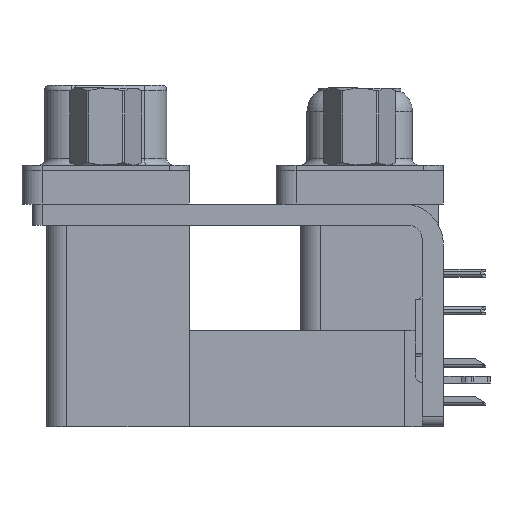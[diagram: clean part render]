
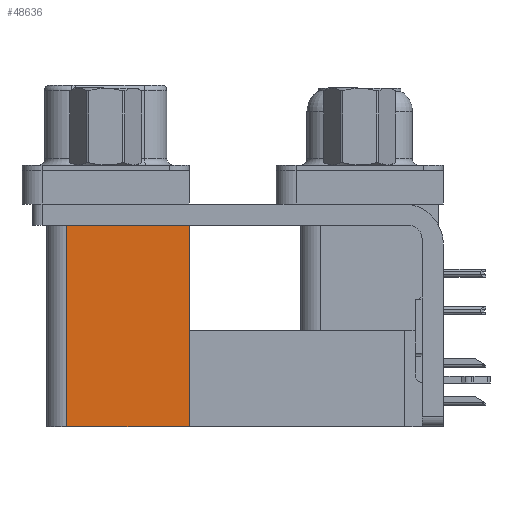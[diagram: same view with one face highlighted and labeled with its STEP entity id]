
A CAD part, left-side view. The second image highlights one B-rep face of the part: STEP entity #48636.
In plain terms, the highlighted planar face has unit normal (-1, 0, 0).
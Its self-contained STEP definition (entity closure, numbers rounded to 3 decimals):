
#2880 = VERTEX_POINT ( 'NONE', #27236 ) ;
#2899 = VECTOR ( 'NONE', #43220, 1000. ) ;
#3665 = PLANE ( 'NONE',  #28769 ) ;
#4022 = EDGE_CURVE ( 'NONE', #26242, #2880, #50487, .T. ) ;
#4644 = ORIENTED_EDGE ( 'NONE', *, *, #35973, .T. ) ;
#4937 = VECTOR ( 'NONE', #23783, 1000. ) ;
#6609 = DIRECTION ( 'NONE',  ( 0., 0., 1. ) ) ;
#11886 = EDGE_CURVE ( 'NONE', #21347, #39069, #47048, .T. ) ;
#13878 = CARTESIAN_POINT ( 'NONE',  ( 3.765, 12.775, -2.5 ) ) ;
#14969 = DIRECTION ( 'NONE',  ( 0., 0., -1. ) ) ;
#15819 = EDGE_LOOP ( 'NONE', ( #25377, #41285, #21533, #4644 ) ) ;
#18465 = EDGE_CURVE ( 'NONE', #2880, #39069, #45353, .T. ) ;
#18502 = VECTOR ( 'NONE', #6609, 1000. ) ;
#19319 = FACE_OUTER_BOUND ( 'NONE', #15819, .T. ) ;
#21347 = VERTEX_POINT ( 'NONE', #13878 ) ;
#21432 = DIRECTION ( 'NONE',  ( 0., 0., 1. ) ) ;
#21477 = CARTESIAN_POINT ( 'NONE',  ( 3.765, 21.975, -19.2 ) ) ;
#21533 = ORIENTED_EDGE ( 'NONE', *, *, #4022, .F. ) ;
#23783 = DIRECTION ( 'NONE',  ( 0., 1., 0. ) ) ;
#25377 = ORIENTED_EDGE ( 'NONE', *, *, #11886, .T. ) ;
#26242 = VERTEX_POINT ( 'NONE', #43727 ) ;
#27236 = CARTESIAN_POINT ( 'NONE',  ( 3.765, 21.975, -19.2 ) ) ;
#27514 = CARTESIAN_POINT ( 'NONE',  ( 3.765, 12.775, -19.2 ) ) ;
#27529 = CARTESIAN_POINT ( 'NONE',  ( 3.765, 12.775, -2.5 ) ) ;
#28769 = AXIS2_PLACEMENT_3D ( 'NONE', #27514, #30862, #14969 ) ;
#29378 = LINE ( 'NONE', #36848, #45960 ) ;
#30862 = DIRECTION ( 'NONE',  ( 1., 0., 0. ) ) ;
#35973 = EDGE_CURVE ( 'NONE', #26242, #21347, #29378, .T. ) ;
#36848 = CARTESIAN_POINT ( 'NONE',  ( 3.765, 12.775, -19.2 ) ) ;
#39069 = VERTEX_POINT ( 'NONE', #41819 ) ;
#41285 = ORIENTED_EDGE ( 'NONE', *, *, #18465, .F. ) ;
#41819 = CARTESIAN_POINT ( 'NONE',  ( 3.765, 21.975, -2.5 ) ) ;
#43220 = DIRECTION ( 'NONE',  ( 0., 1., 0. ) ) ;
#43727 = CARTESIAN_POINT ( 'NONE',  ( 3.765, 12.775, -19.2 ) ) ;
#45353 = LINE ( 'NONE', #21477, #18502 ) ;
#45960 = VECTOR ( 'NONE', #21432, 1000. ) ;
#47048 = LINE ( 'NONE', #27529, #2899 ) ;
#48636 = ADVANCED_FACE ( 'NONE', ( #19319 ), #3665, .F. ) ;
#50240 = CARTESIAN_POINT ( 'NONE',  ( 3.765, 12.775, -19.2 ) ) ;
#50487 = LINE ( 'NONE', #50240, #4937 ) ;
